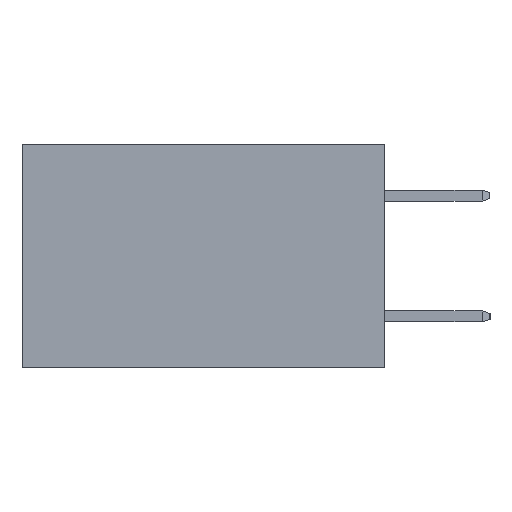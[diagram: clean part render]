
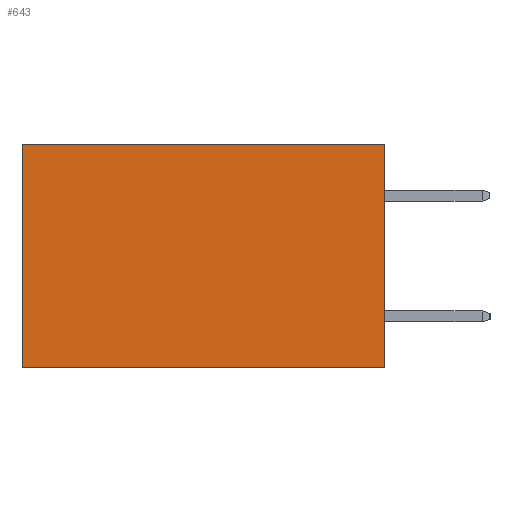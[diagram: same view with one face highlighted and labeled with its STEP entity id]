
A CAD part, left-side view. The second image highlights one B-rep face of the part: STEP entity #643.
In plain terms, the highlighted planar face has unit normal (-1, 0, 0).
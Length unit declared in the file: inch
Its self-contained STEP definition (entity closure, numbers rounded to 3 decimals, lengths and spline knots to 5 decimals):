
#30 = FACE_OUTER_BOUND ( 'NONE', #54, .T. ) ;
#54 = EDGE_LOOP ( 'NONE', ( #5172, #4020, #5825, #9391 ) ) ;
#643 = ADVANCED_FACE ( 'NONE', ( #30 ), #4342, .F. ) ;
#724 = AXIS2_PLACEMENT_3D ( 'NONE', #9690, #4979, #5059 ) ;
#961 = CARTESIAN_POINT ( 'NONE',  ( 0.2615, 0.6, 0. ) ) ;
#1533 = VERTEX_POINT ( 'NONE', #961 ) ;
#2045 = DIRECTION ( 'NONE',  ( 0., 0., -1. ) ) ;
#2118 = CARTESIAN_POINT ( 'NONE',  ( 0.2615, 0.6, -0.37 ) ) ;
#2166 = CARTESIAN_POINT ( 'NONE',  ( 0.2615, 0., -0.37 ) ) ;
#2764 = LINE ( 'NONE', #8619, #4672 ) ;
#2961 = VERTEX_POINT ( 'NONE', #10429 ) ;
#3105 = EDGE_CURVE ( 'NONE', #2961, #1533, #8339, .T. ) ;
#3360 = VERTEX_POINT ( 'NONE', #2166 ) ;
#3369 = EDGE_CURVE ( 'NONE', #1533, #3604, #6923, .T. ) ;
#3604 = VERTEX_POINT ( 'NONE', #9199 ) ;
#4020 = ORIENTED_EDGE ( 'NONE', *, *, #6020, .F. ) ;
#4342 = PLANE ( 'NONE',  #724 ) ;
#4672 = VECTOR ( 'NONE', #8414, 39.37008 ) ;
#4979 = DIRECTION ( 'NONE',  ( 1., 0., 0. ) ) ;
#5059 = DIRECTION ( 'NONE',  ( 0., 0., -1. ) ) ;
#5172 = ORIENTED_EDGE ( 'NONE', *, *, #3369, .T. ) ;
#5825 = ORIENTED_EDGE ( 'NONE', *, *, #6079, .F. ) ;
#6020 = EDGE_CURVE ( 'NONE', #3360, #3604, #2764, .T. ) ;
#6079 = EDGE_CURVE ( 'NONE', #2961, #3360, #8588, .T. ) ;
#6149 = VECTOR ( 'NONE', #6602, 39.37008 ) ;
#6411 = VECTOR ( 'NONE', #8106, 39.37008 ) ;
#6602 = DIRECTION ( 'NONE',  ( 0., 1., 0. ) ) ;
#6807 = CARTESIAN_POINT ( 'NONE',  ( 0.2615, 0., 0. ) ) ;
#6923 = LINE ( 'NONE', #2118, #9280 ) ;
#8094 = CARTESIAN_POINT ( 'NONE',  ( 0.2615, 0., -0.37 ) ) ;
#8106 = DIRECTION ( 'NONE',  ( 0., 0., -1. ) ) ;
#8339 = LINE ( 'NONE', #6807, #6149 ) ;
#8414 = DIRECTION ( 'NONE',  ( 0., 1., 0. ) ) ;
#8588 = LINE ( 'NONE', #8094, #6411 ) ;
#8619 = CARTESIAN_POINT ( 'NONE',  ( 0.2615, 0., -0.37 ) ) ;
#9199 = CARTESIAN_POINT ( 'NONE',  ( 0.2615, 0.6, -0.37 ) ) ;
#9280 = VECTOR ( 'NONE', #2045, 39.37008 ) ;
#9391 = ORIENTED_EDGE ( 'NONE', *, *, #3105, .T. ) ;
#9690 = CARTESIAN_POINT ( 'NONE',  ( 0.2615, 0., -0.37 ) ) ;
#10429 = CARTESIAN_POINT ( 'NONE',  ( 0.2615, 0., 0. ) ) ;
